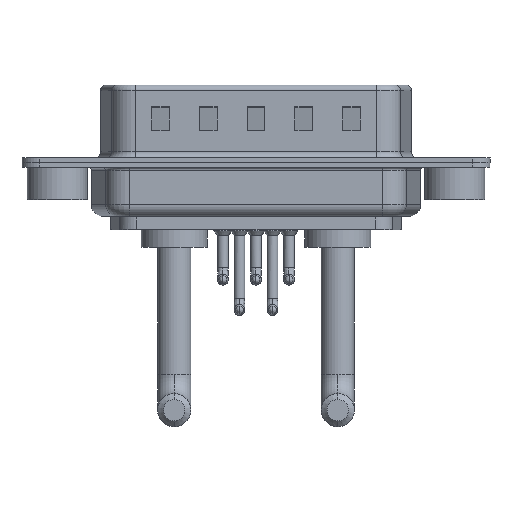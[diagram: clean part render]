
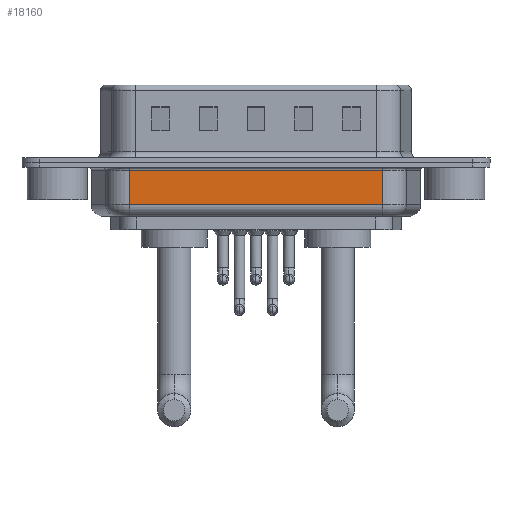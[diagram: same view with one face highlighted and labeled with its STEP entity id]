
A CAD part, front view. The second image highlights one B-rep face of the part: STEP entity #18160.
In plain terms, the highlighted planar face has unit normal (0, -1, 0).
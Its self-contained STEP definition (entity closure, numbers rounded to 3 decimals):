
#175 = DIRECTION ( 'NONE',  ( -1., 0., 0. ) ) ;
#423 = CARTESIAN_POINT ( 'NONE',  ( 6.031, -5.35, -4.5 ) ) ;
#728 = LINE ( 'NONE', #7179, #17120 ) ;
#1814 = LINE ( 'NONE', #423, #12583 ) ;
#2349 = VERTEX_POINT ( 'NONE', #12231 ) ;
#2628 = EDGE_CURVE ( 'NONE', #13914, #2349, #728, .T. ) ;
#2834 = EDGE_CURVE ( 'NONE', #18917, #13914, #14702, .T. ) ;
#3471 = VECTOR ( 'NONE', #20868, 1000. ) ;
#4507 = ORIENTED_EDGE ( 'NONE', *, *, #2628, .T. ) ;
#5232 = CARTESIAN_POINT ( 'NONE',  ( 27.269, -5.35, -3.5 ) ) ;
#5826 = DIRECTION ( 'NONE',  ( 0., 0., 1. ) ) ;
#5930 = VECTOR ( 'NONE', #175, 1000. ) ;
#6016 = DIRECTION ( 'NONE',  ( 0., 0., 1. ) ) ;
#6614 = VERTEX_POINT ( 'NONE', #16474 ) ;
#7179 = CARTESIAN_POINT ( 'NONE',  ( 27.269, -5.35, -4.5 ) ) ;
#7500 = EDGE_CURVE ( 'NONE', #18917, #6614, #1814, .T. ) ;
#7635 = FACE_OUTER_BOUND ( 'NONE', #13422, .T. ) ;
#8208 = ORIENTED_EDGE ( 'NONE', *, *, #10099, .T. ) ;
#8227 = CARTESIAN_POINT ( 'NONE',  ( 6.031, -5.35, -0.65 ) ) ;
#8230 = CARTESIAN_POINT ( 'NONE',  ( 6.031, -5.35, -3.5 ) ) ;
#8269 = DIRECTION ( 'NONE',  ( 0., 0., 1. ) ) ;
#10099 = EDGE_CURVE ( 'NONE', #2349, #6614, #17481, .T. ) ;
#10624 = DIRECTION ( 'NONE',  ( 0., 1., 0. ) ) ;
#10935 = CARTESIAN_POINT ( 'NONE',  ( 6.031, -5.35, -4.5 ) ) ;
#12231 = CARTESIAN_POINT ( 'NONE',  ( 27.269, -5.35, -0.65 ) ) ;
#12583 = VECTOR ( 'NONE', #8269, 1000. ) ;
#13422 = EDGE_LOOP ( 'NONE', ( #14028, #20033, #4507, #8208 ) ) ;
#13914 = VERTEX_POINT ( 'NONE', #5232 ) ;
#14028 = ORIENTED_EDGE ( 'NONE', *, *, #7500, .F. ) ;
#14702 = LINE ( 'NONE', #16198, #3471 ) ;
#16198 = CARTESIAN_POINT ( 'NONE',  ( 6.031, -5.35, -3.5 ) ) ;
#16474 = CARTESIAN_POINT ( 'NONE',  ( 6.031, -5.35, -0.65 ) ) ;
#17120 = VECTOR ( 'NONE', #6016, 1000. ) ;
#17203 = PLANE ( 'NONE',  #18892 ) ;
#17481 = LINE ( 'NONE', #8227, #5930 ) ;
#18160 = ADVANCED_FACE ( 'NONE', ( #7635 ), #17203, .F. ) ;
#18892 = AXIS2_PLACEMENT_3D ( 'NONE', #10935, #10624, #5826 ) ;
#18917 = VERTEX_POINT ( 'NONE', #8230 ) ;
#20033 = ORIENTED_EDGE ( 'NONE', *, *, #2834, .T. ) ;
#20868 = DIRECTION ( 'NONE',  ( 1., 0., 0. ) ) ;
